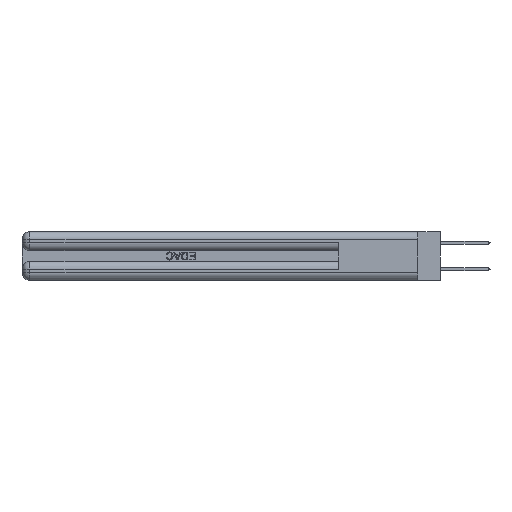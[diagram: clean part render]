
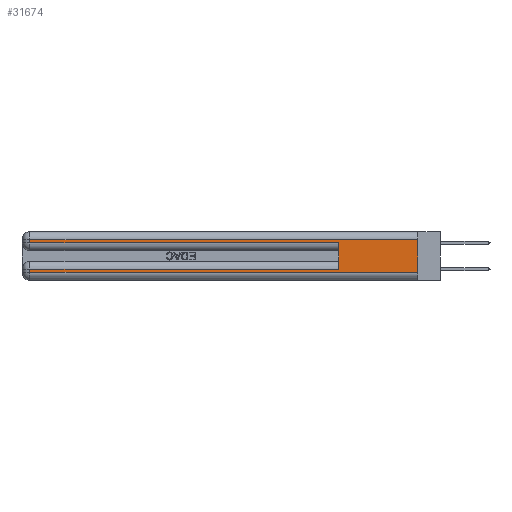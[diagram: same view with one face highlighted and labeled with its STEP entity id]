
A CAD part, left-side view. The second image highlights one B-rep face of the part: STEP entity #31674.
In plain terms, the highlighted planar face has unit normal (-1, 0, 0).
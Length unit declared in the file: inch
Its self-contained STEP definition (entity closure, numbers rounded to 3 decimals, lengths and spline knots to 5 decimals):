
#225 = VECTOR ( 'NONE', #23291, 39.37008 ) ;
#278 = DIRECTION ( 'NONE',  ( 0., -1., 0. ) ) ;
#756 = CARTESIAN_POINT ( 'NONE',  ( 0., 0.6, 0.085 ) ) ;
#1366 = CARTESIAN_POINT ( 'NONE',  ( 0., 0., 0.37 ) ) ;
#2124 = EDGE_CURVE ( 'NONE', #14071, #2640, #23739, .T. ) ;
#2640 = VERTEX_POINT ( 'NONE', #20701 ) ;
#2970 = VECTOR ( 'NONE', #31559, 39.37008 ) ;
#3028 = CARTESIAN_POINT ( 'NONE',  ( 0., 2.94, 0.37 ) ) ;
#3090 = CARTESIAN_POINT ( 'NONE',  ( 0., 2.94, 0.37 ) ) ;
#3778 = DIRECTION ( 'NONE',  ( 0., 1., 0. ) ) ;
#4363 = CARTESIAN_POINT ( 'NONE',  ( 0., 2.94, 0.06 ) ) ;
#4764 = VERTEX_POINT ( 'NONE', #4363 ) ;
#5806 = VECTOR ( 'NONE', #18075, 39.37008 ) ;
#6648 = DIRECTION ( 'NONE',  ( 0., 0., -1. ) ) ;
#6885 = EDGE_CURVE ( 'NONE', #10581, #32979, #43807, .T. ) ;
#7252 = CARTESIAN_POINT ( 'NONE',  ( 0., 0., 0.31 ) ) ;
#8003 = EDGE_CURVE ( 'NONE', #8624, #4764, #21988, .T. ) ;
#8091 = EDGE_LOOP ( 'NONE', ( #9149, #32105, #30446, #16434, #46047, #35191, #27244, #29596 ) ) ;
#8624 = VERTEX_POINT ( 'NONE', #21287 ) ;
#8776 = VECTOR ( 'NONE', #6648, 39.37008 ) ;
#9149 = ORIENTED_EDGE ( 'NONE', *, *, #19795, .F. ) ;
#9712 = VERTEX_POINT ( 'NONE', #40721 ) ;
#10581 = VERTEX_POINT ( 'NONE', #756 ) ;
#11469 = CARTESIAN_POINT ( 'NONE',  ( 0., 0., 0.37 ) ) ;
#14000 = EDGE_CURVE ( 'NONE', #4764, #9712, #28753, .T. ) ;
#14071 = VERTEX_POINT ( 'NONE', #30872 ) ;
#15764 = PLANE ( 'NONE',  #35619 ) ;
#16371 = EDGE_CURVE ( 'NONE', #2640, #34200, #37178, .T. ) ;
#16434 = ORIENTED_EDGE ( 'NONE', *, *, #30683, .T. ) ;
#16714 = FACE_OUTER_BOUND ( 'NONE', #8091, .T. ) ;
#18075 = DIRECTION ( 'NONE',  ( 0., 1., 0. ) ) ;
#18979 = VECTOR ( 'NONE', #3778, 39.37008 ) ;
#19345 = DIRECTION ( 'NONE',  ( 0., 0., -1. ) ) ;
#19695 = CARTESIAN_POINT ( 'NONE',  ( 0., 0., 0.06 ) ) ;
#19795 = EDGE_CURVE ( 'NONE', #14071, #9712, #36932, .T. ) ;
#20701 = CARTESIAN_POINT ( 'NONE',  ( 0., 2.94, 0.31 ) ) ;
#21287 = CARTESIAN_POINT ( 'NONE',  ( 0., 2.94, 0.085 ) ) ;
#21297 = VECTOR ( 'NONE', #278, 39.37008 ) ;
#21432 = CARTESIAN_POINT ( 'NONE',  ( 0., 2.94, 0.285 ) ) ;
#21988 = LINE ( 'NONE', #3028, #2970 ) ;
#22748 = EDGE_CURVE ( 'NONE', #10581, #8624, #29583, .T. ) ;
#23291 = DIRECTION ( 'NONE',  ( 0., -1., 0. ) ) ;
#23739 = LINE ( 'NONE', #7252, #5806 ) ;
#25179 = CARTESIAN_POINT ( 'NONE',  ( 0., 0., 0.085 ) ) ;
#25286 = CARTESIAN_POINT ( 'NONE',  ( 0., 0., 0.285 ) ) ;
#27244 = ORIENTED_EDGE ( 'NONE', *, *, #8003, .T. ) ;
#28753 = LINE ( 'NONE', #19695, #225 ) ;
#29583 = LINE ( 'NONE', #25179, #18979 ) ;
#29596 = ORIENTED_EDGE ( 'NONE', *, *, #14000, .T. ) ;
#30446 = ORIENTED_EDGE ( 'NONE', *, *, #16371, .T. ) ;
#30683 = EDGE_CURVE ( 'NONE', #34200, #32979, #30727, .T. ) ;
#30727 = LINE ( 'NONE', #25286, #21297 ) ;
#30872 = CARTESIAN_POINT ( 'NONE',  ( 0., 0., 0.31 ) ) ;
#31559 = DIRECTION ( 'NONE',  ( 0., 0., -1. ) ) ;
#31674 = ADVANCED_FACE ( 'NONE', ( #16714 ), #15764, .F. ) ;
#32105 = ORIENTED_EDGE ( 'NONE', *, *, #2124, .T. ) ;
#32891 = CARTESIAN_POINT ( 'NONE',  ( 0., 0.6, 0.145 ) ) ;
#32979 = VERTEX_POINT ( 'NONE', #41406 ) ;
#34200 = VERTEX_POINT ( 'NONE', #21432 ) ;
#35191 = ORIENTED_EDGE ( 'NONE', *, *, #22748, .T. ) ;
#35619 = AXIS2_PLACEMENT_3D ( 'NONE', #1366, #40586, #19345 ) ;
#36932 = LINE ( 'NONE', #11469, #45227 ) ;
#37178 = LINE ( 'NONE', #3090, #8776 ) ;
#40021 = DIRECTION ( 'NONE',  ( 0., 0., -1. ) ) ;
#40586 = DIRECTION ( 'NONE',  ( 1., 0., 0. ) ) ;
#40721 = CARTESIAN_POINT ( 'NONE',  ( 0., 0., 0.06 ) ) ;
#41406 = CARTESIAN_POINT ( 'NONE',  ( 0., 0.6, 0.285 ) ) ;
#42695 = VECTOR ( 'NONE', #43390, 39.37008 ) ;
#43390 = DIRECTION ( 'NONE',  ( 0., 0., 1. ) ) ;
#43807 = LINE ( 'NONE', #32891, #42695 ) ;
#45227 = VECTOR ( 'NONE', #40021, 39.37008 ) ;
#46047 = ORIENTED_EDGE ( 'NONE', *, *, #6885, .F. ) ;
